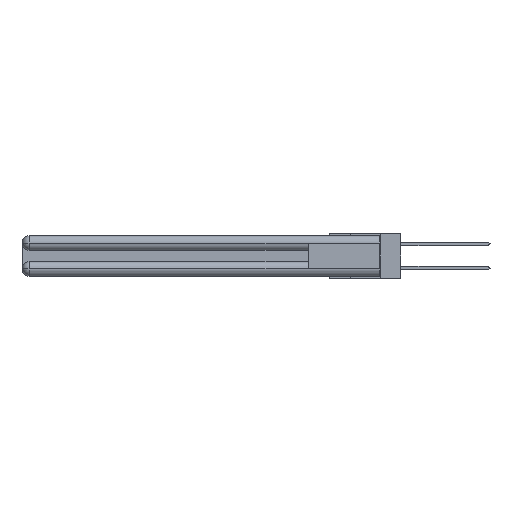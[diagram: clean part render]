
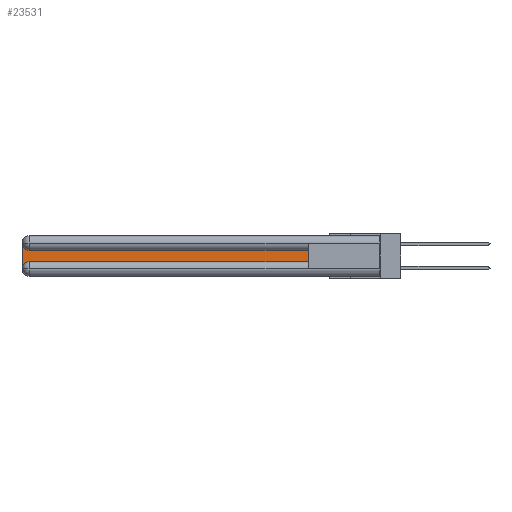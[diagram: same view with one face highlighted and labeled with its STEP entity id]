
A CAD part, left-side view. The second image highlights one B-rep face of the part: STEP entity #23531.
In plain terms, the highlighted planar face has unit normal (-1, 0, 0).
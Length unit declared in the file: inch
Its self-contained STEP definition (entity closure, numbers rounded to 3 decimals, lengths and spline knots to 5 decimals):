
#273 = AXIS2_PLACEMENT_3D ( 'NONE', #2099, #26080, #2215 ) ;
#1047 = EDGE_CURVE ( 'NONE', #22860, #14363, #7251, .T. ) ;
#1323 = VERTEX_POINT ( 'NONE', #7620 ) ;
#1420 = CARTESIAN_POINT ( 'NONE',  ( 0.075, 2.94, -0.2175 ) ) ;
#2099 = CARTESIAN_POINT ( 'NONE',  ( 0.075, 3., -0.1225 ) ) ;
#2215 = DIRECTION ( 'NONE',  ( 0., 0., -1. ) ) ;
#2221 = EDGE_CURVE ( 'NONE', #30059, #1323, #23885, .T. ) ;
#4178 = DIRECTION ( 'NONE',  ( 0., 0., 1. ) ) ;
#4379 = ORIENTED_EDGE ( 'NONE', *, *, #17603, .T. ) ;
#4861 = LINE ( 'NONE', #14268, #18260 ) ;
#5299 = DIRECTION ( 'NONE',  ( 0., 0., -1. ) ) ;
#5307 = EDGE_CURVE ( 'NONE', #1323, #24366, #16326, .T. ) ;
#7251 = LINE ( 'NONE', #29615, #34407 ) ;
#7620 = CARTESIAN_POINT ( 'NONE',  ( 0.075, 0.6, -0.2175 ) ) ;
#8939 = DIRECTION ( 'NONE',  ( 0., 0., -1. ) ) ;
#10252 = EDGE_CURVE ( 'NONE', #11639, #22860, #26112, .T. ) ;
#10258 = CARTESIAN_POINT ( 'NONE',  ( 0.075, 3., -0.0625 ) ) ;
#10834 = VECTOR ( 'NONE', #4178, 39.37008 ) ;
#10902 = FACE_OUTER_BOUND ( 'NONE', #34079, .T. ) ;
#11639 = VERTEX_POINT ( 'NONE', #31432 ) ;
#11943 = DIRECTION ( 'NONE',  ( 0., -1., 0. ) ) ;
#13485 = ORIENTED_EDGE ( 'NONE', *, *, #1047, .T. ) ;
#14268 = CARTESIAN_POINT ( 'NONE',  ( 0.075, 0.6, -0.1225 ) ) ;
#14363 = VERTEX_POINT ( 'NONE', #26576 ) ;
#14473 = CARTESIAN_POINT ( 'NONE',  ( 0.075, 2.94, -0.0625 ) ) ;
#15593 = EDGE_CURVE ( 'NONE', #24366, #11639, #4861, .T. ) ;
#16326 = LINE ( 'NONE', #17172, #10834 ) ;
#17172 = CARTESIAN_POINT ( 'NONE',  ( 0.075, 0.6, -0.2175 ) ) ;
#17603 = EDGE_CURVE ( 'NONE', #14363, #30059, #28274, .T. ) ;
#18260 = VECTOR ( 'NONE', #32874, 39.37008 ) ;
#20637 = ORIENTED_EDGE ( 'NONE', *, *, #15593, .T. ) ;
#22860 = VERTEX_POINT ( 'NONE', #10258 ) ;
#23497 = ORIENTED_EDGE ( 'NONE', *, *, #2221, .T. ) ;
#23531 = ADVANCED_FACE ( 'NONE', ( #10902 ), #34488, .F. ) ;
#23885 = LINE ( 'NONE', #25143, #29300 ) ;
#24366 = VERTEX_POINT ( 'NONE', #31876 ) ;
#25143 = CARTESIAN_POINT ( 'NONE',  ( 0.075, 0.6, -0.2175 ) ) ;
#25883 = AXIS2_PLACEMENT_3D ( 'NONE', #26401, #31542, #26514 ) ;
#26080 = DIRECTION ( 'NONE',  ( 1., 0., 0. ) ) ;
#26112 = CIRCLE ( 'NONE', #28858, 0.06 ) ;
#26401 = CARTESIAN_POINT ( 'NONE',  ( 0.075, 2.94, -0.2775 ) ) ;
#26514 = DIRECTION ( 'NONE',  ( 0., 0., -1. ) ) ;
#26576 = CARTESIAN_POINT ( 'NONE',  ( 0.075, 3., -0.2775 ) ) ;
#28274 = CIRCLE ( 'NONE', #25883, 0.06 ) ;
#28858 = AXIS2_PLACEMENT_3D ( 'NONE', #14473, #30538, #8939 ) ;
#29300 = VECTOR ( 'NONE', #11943, 39.37008 ) ;
#29615 = CARTESIAN_POINT ( 'NONE',  ( 0.075, 3., -0.2175 ) ) ;
#29728 = ORIENTED_EDGE ( 'NONE', *, *, #10252, .T. ) ;
#30059 = VERTEX_POINT ( 'NONE', #1420 ) ;
#30538 = DIRECTION ( 'NONE',  ( 1., 0., 0. ) ) ;
#31432 = CARTESIAN_POINT ( 'NONE',  ( 0.075, 2.94, -0.1225 ) ) ;
#31542 = DIRECTION ( 'NONE',  ( 1., 0., 0. ) ) ;
#31876 = CARTESIAN_POINT ( 'NONE',  ( 0.075, 0.6, -0.1225 ) ) ;
#32606 = ORIENTED_EDGE ( 'NONE', *, *, #5307, .T. ) ;
#32874 = DIRECTION ( 'NONE',  ( 0., 1., 0. ) ) ;
#34079 = EDGE_LOOP ( 'NONE', ( #20637, #29728, #13485, #4379, #23497, #32606 ) ) ;
#34407 = VECTOR ( 'NONE', #5299, 39.37008 ) ;
#34488 = PLANE ( 'NONE',  #273 ) ;
